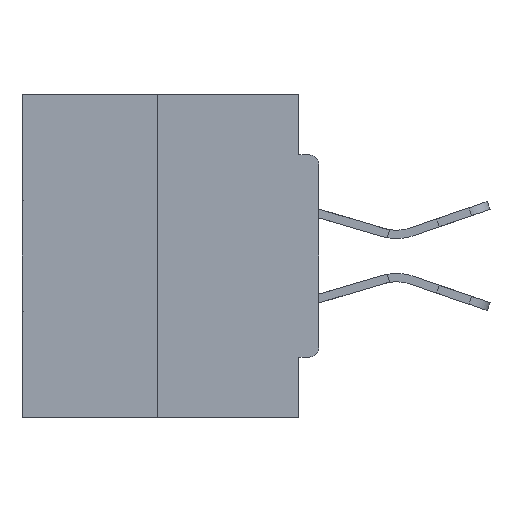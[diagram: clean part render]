
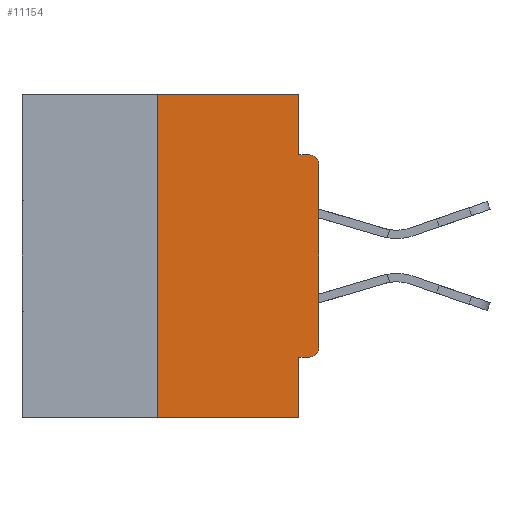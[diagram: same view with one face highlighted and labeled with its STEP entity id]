
A CAD part, left-side view. The second image highlights one B-rep face of the part: STEP entity #11154.
In plain terms, the highlighted planar face has unit normal (-1, 0, 0).
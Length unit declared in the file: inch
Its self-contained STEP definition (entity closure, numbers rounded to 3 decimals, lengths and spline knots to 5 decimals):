
#568 = DIRECTION ( 'NONE',  ( 1., 0., 0. ) ) ;
#711 = CARTESIAN_POINT ( 'NONE',  ( 0., 0.015, -0.3915 ) ) ;
#742 = CIRCLE ( 'NONE', #31635, 0.015 ) ;
#1277 = ORIENTED_EDGE ( 'NONE', *, *, #15750, .F. ) ;
#2244 = VERTEX_POINT ( 'NONE', #28119 ) ;
#2335 = DIRECTION ( 'NONE',  ( 0., 1., 0. ) ) ;
#2826 = CARTESIAN_POINT ( 'NONE',  ( 0., 0., -0.0935 ) ) ;
#3015 = CARTESIAN_POINT ( 'NONE',  ( 0., 0.46, -0.5 ) ) ;
#3090 = EDGE_CURVE ( 'NONE', #11405, #11672, #34069, .T. ) ;
#3703 = DIRECTION ( 'NONE',  ( -1., 0., 0. ) ) ;
#3829 = CIRCLE ( 'NONE', #15345, 0.015 ) ;
#4043 = ORIENTED_EDGE ( 'NONE', *, *, #24143, .T. ) ;
#4067 = CARTESIAN_POINT ( 'NONE',  ( 0., 0.015, -0.1085 ) ) ;
#5551 = LINE ( 'NONE', #23466, #19894 ) ;
#6067 = ORIENTED_EDGE ( 'NONE', *, *, #15258, .F. ) ;
#6190 = CARTESIAN_POINT ( 'NONE',  ( 0., 0.031, -0.5 ) ) ;
#6363 = VECTOR ( 'NONE', #12909, 39.37008 ) ;
#6425 = EDGE_CURVE ( 'NONE', #16790, #27204, #14481, .T. ) ;
#6655 = ORIENTED_EDGE ( 'NONE', *, *, #11857, .F. ) ;
#6921 = DIRECTION ( 'NONE',  ( 0., 0., -1. ) ) ;
#6997 = VECTOR ( 'NONE', #20180, 39.37008 ) ;
#8683 = CARTESIAN_POINT ( 'NONE',  ( 0., 0.031, -0.0935 ) ) ;
#9244 = DIRECTION ( 'NONE',  ( 0., -1., 0. ) ) ;
#9830 = VERTEX_POINT ( 'NONE', #11617 ) ;
#10078 = DIRECTION ( 'NONE',  ( -1., 0., 0. ) ) ;
#10294 = DIRECTION ( 'NONE',  ( 0., 0., -1. ) ) ;
#11154 = ADVANCED_FACE ( 'NONE', ( #13006 ), #25114, .F. ) ;
#11316 = CARTESIAN_POINT ( 'NONE',  ( 0., 0.25, 0. ) ) ;
#11405 = VERTEX_POINT ( 'NONE', #27097 ) ;
#11617 = CARTESIAN_POINT ( 'NONE',  ( 0., 0., -0.1085 ) ) ;
#11672 = VERTEX_POINT ( 'NONE', #28506 ) ;
#11844 = EDGE_CURVE ( 'NONE', #2244, #17694, #27809, .T. ) ;
#11857 = EDGE_CURVE ( 'NONE', #11672, #16790, #20752, .T. ) ;
#12005 = ORIENTED_EDGE ( 'NONE', *, *, #36055, .F. ) ;
#12909 = DIRECTION ( 'NONE',  ( 0., 0., -1. ) ) ;
#12924 = EDGE_CURVE ( 'NONE', #13538, #28094, #3829, .T. ) ;
#13006 = FACE_OUTER_BOUND ( 'NONE', #25478, .T. ) ;
#13048 = DIRECTION ( 'NONE',  ( 0., -1., 0. ) ) ;
#13189 = CARTESIAN_POINT ( 'NONE',  ( 0., 0.46, 0. ) ) ;
#13538 = VERTEX_POINT ( 'NONE', #21072 ) ;
#14481 = LINE ( 'NONE', #2826, #17109 ) ;
#14649 = VECTOR ( 'NONE', #15286, 39.37008 ) ;
#15258 = EDGE_CURVE ( 'NONE', #13538, #31569, #5551, .T. ) ;
#15286 = DIRECTION ( 'NONE',  ( 0., 0., -1. ) ) ;
#15345 = AXIS2_PLACEMENT_3D ( 'NONE', #711, #3703, #6921 ) ;
#15750 = EDGE_CURVE ( 'NONE', #2244, #11405, #36346, .T. ) ;
#16310 = LINE ( 'NONE', #28632, #6363 ) ;
#16766 = CARTESIAN_POINT ( 'NONE',  ( 0., 0., 0. ) ) ;
#16790 = VERTEX_POINT ( 'NONE', #8683 ) ;
#16986 = CARTESIAN_POINT ( 'NONE',  ( 0., 0., -0.3915 ) ) ;
#17109 = VECTOR ( 'NONE', #27381, 39.37008 ) ;
#17694 = VERTEX_POINT ( 'NONE', #6190 ) ;
#18899 = CARTESIAN_POINT ( 'NONE',  ( 0., 0.46, 0. ) ) ;
#19894 = VECTOR ( 'NONE', #2335, 39.37008 ) ;
#20180 = DIRECTION ( 'NONE',  ( 0., 0., 1. ) ) ;
#20752 = LINE ( 'NONE', #33864, #14649 ) ;
#21072 = CARTESIAN_POINT ( 'NONE',  ( 0., 0.015, -0.4065 ) ) ;
#22924 = ORIENTED_EDGE ( 'NONE', *, *, #6425, .F. ) ;
#23466 = CARTESIAN_POINT ( 'NONE',  ( 0., 0., -0.4065 ) ) ;
#24143 = EDGE_CURVE ( 'NONE', #9830, #27204, #742, .T. ) ;
#25114 = PLANE ( 'NONE',  #39718 ) ;
#25292 = DIRECTION ( 'NONE',  ( 0., 0., -1. ) ) ;
#25478 = EDGE_LOOP ( 'NONE', ( #30678, #1277, #38789, #12005, #6067, #27558, #29560, #4043, #22924, #6655 ) ) ;
#26048 = VECTOR ( 'NONE', #13048, 39.37008 ) ;
#26370 = VECTOR ( 'NONE', #35972, 39.37008 ) ;
#27097 = CARTESIAN_POINT ( 'NONE',  ( 0., 0.25, 0. ) ) ;
#27204 = VERTEX_POINT ( 'NONE', #29215 ) ;
#27381 = DIRECTION ( 'NONE',  ( 0., -1., 0. ) ) ;
#27558 = ORIENTED_EDGE ( 'NONE', *, *, #12924, .T. ) ;
#27809 = LINE ( 'NONE', #3015, #32080 ) ;
#28094 = VERTEX_POINT ( 'NONE', #16986 ) ;
#28119 = CARTESIAN_POINT ( 'NONE',  ( 0., 0.25, -0.5 ) ) ;
#28506 = CARTESIAN_POINT ( 'NONE',  ( 0., 0.031, 0. ) ) ;
#28632 = CARTESIAN_POINT ( 'NONE',  ( 0., 0.031, -0.5 ) ) ;
#28881 = LINE ( 'NONE', #16766, #6997 ) ;
#29215 = CARTESIAN_POINT ( 'NONE',  ( 0., 0.015, -0.0935 ) ) ;
#29560 = ORIENTED_EDGE ( 'NONE', *, *, #35635, .T. ) ;
#30359 = CARTESIAN_POINT ( 'NONE',  ( 0., 0.031, -0.4065 ) ) ;
#30678 = ORIENTED_EDGE ( 'NONE', *, *, #3090, .F. ) ;
#31569 = VERTEX_POINT ( 'NONE', #30359 ) ;
#31635 = AXIS2_PLACEMENT_3D ( 'NONE', #4067, #10078, #10294 ) ;
#32080 = VECTOR ( 'NONE', #9244, 39.37008 ) ;
#33864 = CARTESIAN_POINT ( 'NONE',  ( 0., 0.031, 0. ) ) ;
#34069 = LINE ( 'NONE', #18899, #26048 ) ;
#35635 = EDGE_CURVE ( 'NONE', #28094, #9830, #28881, .T. ) ;
#35972 = DIRECTION ( 'NONE',  ( 0., 0., 1. ) ) ;
#36055 = EDGE_CURVE ( 'NONE', #31569, #17694, #16310, .T. ) ;
#36346 = LINE ( 'NONE', #11316, #26370 ) ;
#38789 = ORIENTED_EDGE ( 'NONE', *, *, #11844, .T. ) ;
#39718 = AXIS2_PLACEMENT_3D ( 'NONE', #13189, #568, #25292 ) ;
